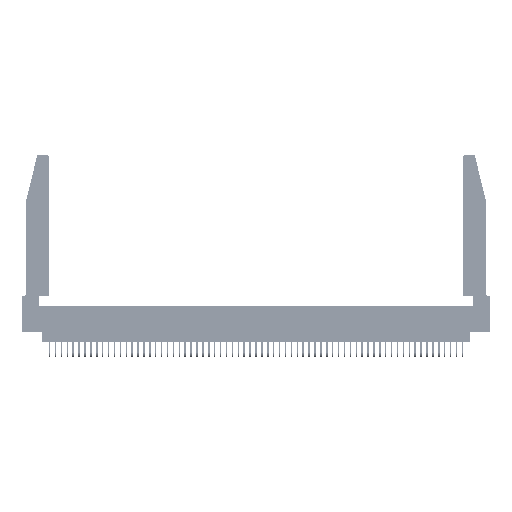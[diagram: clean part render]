
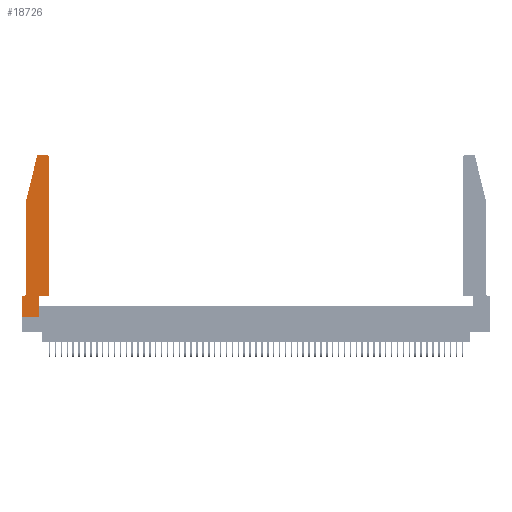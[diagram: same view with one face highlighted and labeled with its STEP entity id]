
A CAD part, top view. The second image highlights one B-rep face of the part: STEP entity #18726.
In plain terms, the highlighted planar face has unit normal (0, 0, 1).
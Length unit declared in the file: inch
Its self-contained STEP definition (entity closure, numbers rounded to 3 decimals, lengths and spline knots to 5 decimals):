
#139 = CARTESIAN_POINT ( 'NONE',  ( 0.2865, 0.35, 0.37 ) ) ;
#305 = DIRECTION ( 'NONE',  ( -1., 0., 0. ) ) ;
#316 = ORIENTED_EDGE ( 'NONE', *, *, #42979, .T. ) ;
#4571 = VERTEX_POINT ( 'NONE', #49980 ) ;
#4602 = LINE ( 'NONE', #5673, #29985 ) ;
#5197 = CARTESIAN_POINT ( 'NONE',  ( 0., 0., 0.37 ) ) ;
#5253 = VECTOR ( 'NONE', #52570, 39.37008 ) ;
#5415 = CARTESIAN_POINT ( 'NONE',  ( 0.4505, 0.35, 0.37 ) ) ;
#5673 = CARTESIAN_POINT ( 'NONE',  ( 0., 0., 0.37 ) ) ;
#6563 = ORIENTED_EDGE ( 'NONE', *, *, #24232, .T. ) ;
#6639 = VERTEX_POINT ( 'NONE', #44622 ) ;
#6791 = CARTESIAN_POINT ( 'NONE',  ( 0.0755, 2., 0.37 ) ) ;
#6937 = CIRCLE ( 'NONE', #10763, 0.03 ) ;
#8934 = ORIENTED_EDGE ( 'NONE', *, *, #36583, .T. ) ;
#9657 = LINE ( 'NONE', #52969, #56068 ) ;
#10116 = EDGE_CURVE ( 'NONE', #31265, #55660, #37147, .T. ) ;
#10231 = DIRECTION ( 'NONE',  ( 0., -1., 0. ) ) ;
#10451 = ORIENTED_EDGE ( 'NONE', *, *, #43793, .T. ) ;
#10743 = CIRCLE ( 'NONE', #23771, 0.03 ) ;
#10763 = AXIS2_PLACEMENT_3D ( 'NONE', #26294, #57691, #30819 ) ;
#11506 = VERTEX_POINT ( 'NONE', #50540 ) ;
#12063 = CARTESIAN_POINT ( 'NONE',  ( 0., 0., 0.37 ) ) ;
#12200 = CARTESIAN_POINT ( 'NONE',  ( 0.0755, 2., 0.37 ) ) ;
#13164 = VECTOR ( 'NONE', #14509, 39.37008 ) ;
#13215 = EDGE_CURVE ( 'NONE', #4571, #31265, #22100, .T. ) ;
#13633 = DIRECTION ( 'NONE',  ( 0., 1., 0. ) ) ;
#14509 = DIRECTION ( 'NONE',  ( 1., 0., 0. ) ) ;
#16402 = CARTESIAN_POINT ( 'NONE',  ( 0.2605, 2.75, 0.37 ) ) ;
#16700 = VERTEX_POINT ( 'NONE', #12200 ) ;
#18726 = ADVANCED_FACE ( 'NONE', ( #52714 ), #42467, .T. ) ;
#19570 = VECTOR ( 'NONE', #51095, 39.37008 ) ;
#19698 = CARTESIAN_POINT ( 'NONE',  ( 0.0755, 0.35, 0.37 ) ) ;
#20114 = CIRCLE ( 'NONE', #39776, 0.07 ) ;
#21698 = ORIENTED_EDGE ( 'NONE', *, *, #29266, .T. ) ;
#21801 = CARTESIAN_POINT ( 'NONE',  ( 0.0755, 0.42, 0.37 ) ) ;
#21803 = EDGE_CURVE ( 'NONE', #55660, #11506, #56546, .T. ) ;
#22100 = LINE ( 'NONE', #53816, #44564 ) ;
#22465 = EDGE_CURVE ( 'NONE', #11506, #6639, #10743, .T. ) ;
#23259 = DIRECTION ( 'NONE',  ( 0., 0., 1. ) ) ;
#23771 = AXIS2_PLACEMENT_3D ( 'NONE', #50152, #23259, #54672 ) ;
#24232 = EDGE_CURVE ( 'NONE', #6639, #42906, #52331, .T. ) ;
#24348 = ORIENTED_EDGE ( 'NONE', *, *, #38615, .T. ) ;
#24457 = EDGE_LOOP ( 'NONE', ( #6563, #34312, #316, #24348, #41409, #8934, #10451, #21698, #26388, #54949, #46038, #36560 ) ) ;
#24608 = DIRECTION ( 'NONE',  ( 1., 0., 0. ) ) ;
#26294 = CARTESIAN_POINT ( 'NONE',  ( 0.284, 2.72, 0.37 ) ) ;
#26388 = ORIENTED_EDGE ( 'NONE', *, *, #13215, .T. ) ;
#27405 = DIRECTION ( 'NONE',  ( 0., 0., -1. ) ) ;
#28405 = VECTOR ( 'NONE', #43662, 39.37008 ) ;
#29266 = EDGE_CURVE ( 'NONE', #56944, #4571, #41189, .T. ) ;
#29985 = VECTOR ( 'NONE', #10231, 39.37008 ) ;
#30819 = DIRECTION ( 'NONE',  ( 1., 0., 0. ) ) ;
#31104 = EDGE_CURVE ( 'NONE', #42906, #31869, #6937, .T. ) ;
#31265 = VERTEX_POINT ( 'NONE', #139 ) ;
#31534 = CARTESIAN_POINT ( 'NONE',  ( 0.25487, 2.72718, 0.37 ) ) ;
#31869 = VERTEX_POINT ( 'NONE', #31534 ) ;
#32902 = LINE ( 'NONE', #19698, #19570 ) ;
#34312 = ORIENTED_EDGE ( 'NONE', *, *, #31104, .T. ) ;
#35344 = DIRECTION ( 'NONE',  ( -0.239, -0.971, 0. ) ) ;
#35424 = VERTEX_POINT ( 'NONE', #56836 ) ;
#36560 = ORIENTED_EDGE ( 'NONE', *, *, #22465, .T. ) ;
#36583 = EDGE_CURVE ( 'NONE', #35424, #49845, #32902, .T. ) ;
#37147 = LINE ( 'NONE', #5415, #13164 ) ;
#38615 = EDGE_CURVE ( 'NONE', #16700, #50533, #57205, .T. ) ;
#39776 = AXIS2_PLACEMENT_3D ( 'NONE', #54338, #27405, #305 ) ;
#40580 = CARTESIAN_POINT ( 'NONE',  ( 0.4505, 0.35, 0.37 ) ) ;
#41189 = LINE ( 'NONE', #12063, #5253 ) ;
#41409 = ORIENTED_EDGE ( 'NONE', *, *, #57417, .T. ) ;
#42467 = PLANE ( 'NONE',  #53296 ) ;
#42906 = VERTEX_POINT ( 'NONE', #43750 ) ;
#42979 = EDGE_CURVE ( 'NONE', #31869, #16700, #9657, .T. ) ;
#43662 = DIRECTION ( 'NONE',  ( -1., 0., 0. ) ) ;
#43750 = CARTESIAN_POINT ( 'NONE',  ( 0.284, 2.75, 0.37 ) ) ;
#43793 = EDGE_CURVE ( 'NONE', #49845, #56944, #4602, .T. ) ;
#44564 = VECTOR ( 'NONE', #58290, 39.37008 ) ;
#44621 = VECTOR ( 'NONE', #13633, 39.37008 ) ;
#44622 = CARTESIAN_POINT ( 'NONE',  ( 0.4205, 2.75, 0.37 ) ) ;
#45693 = CARTESIAN_POINT ( 'NONE',  ( 0.4505, 0.35, 0.37 ) ) ;
#46038 = ORIENTED_EDGE ( 'NONE', *, *, #21803, .T. ) ;
#46989 = CARTESIAN_POINT ( 'NONE',  ( 0., 0.35, 0.37 ) ) ;
#49845 = VERTEX_POINT ( 'NONE', #57755 ) ;
#49980 = CARTESIAN_POINT ( 'NONE',  ( 0.2865, 0., 0.37 ) ) ;
#50152 = CARTESIAN_POINT ( 'NONE',  ( 0.4205, 2.72, 0.37 ) ) ;
#50533 = VERTEX_POINT ( 'NONE', #21801 ) ;
#50540 = CARTESIAN_POINT ( 'NONE',  ( 0.4505, 2.72, 0.37 ) ) ;
#51095 = DIRECTION ( 'NONE',  ( -1., 0., 0. ) ) ;
#51517 = DIRECTION ( 'NONE',  ( 0., 0., 1. ) ) ;
#52331 = LINE ( 'NONE', #16402, #28405 ) ;
#52570 = DIRECTION ( 'NONE',  ( 1., 0., 0. ) ) ;
#52714 = FACE_OUTER_BOUND ( 'NONE', #24457, .T. ) ;
#52969 = CARTESIAN_POINT ( 'NONE',  ( 0.0755, 2., 0.37 ) ) ;
#53296 = AXIS2_PLACEMENT_3D ( 'NONE', #46989, #51517, #24608 ) ;
#53816 = CARTESIAN_POINT ( 'NONE',  ( 0.2865, 0.35, 0.37 ) ) ;
#54338 = CARTESIAN_POINT ( 'NONE',  ( 0.0055, 0.42, 0.37 ) ) ;
#54672 = DIRECTION ( 'NONE',  ( 1., 0., 0. ) ) ;
#54949 = ORIENTED_EDGE ( 'NONE', *, *, #10116, .T. ) ;
#55660 = VERTEX_POINT ( 'NONE', #45693 ) ;
#55815 = VECTOR ( 'NONE', #56159, 39.37008 ) ;
#56068 = VECTOR ( 'NONE', #35344, 39.37008 ) ;
#56159 = DIRECTION ( 'NONE',  ( 0., -1., 0. ) ) ;
#56546 = LINE ( 'NONE', #40580, #44621 ) ;
#56836 = CARTESIAN_POINT ( 'NONE',  ( 0.0055, 0.35, 0.37 ) ) ;
#56944 = VERTEX_POINT ( 'NONE', #5197 ) ;
#57205 = LINE ( 'NONE', #6791, #55815 ) ;
#57417 = EDGE_CURVE ( 'NONE', #50533, #35424, #20114, .T. ) ;
#57691 = DIRECTION ( 'NONE',  ( 0., 0., 1. ) ) ;
#57755 = CARTESIAN_POINT ( 'NONE',  ( 0., 0.35, 0.37 ) ) ;
#58290 = DIRECTION ( 'NONE',  ( 0., 1., 0. ) ) ;
